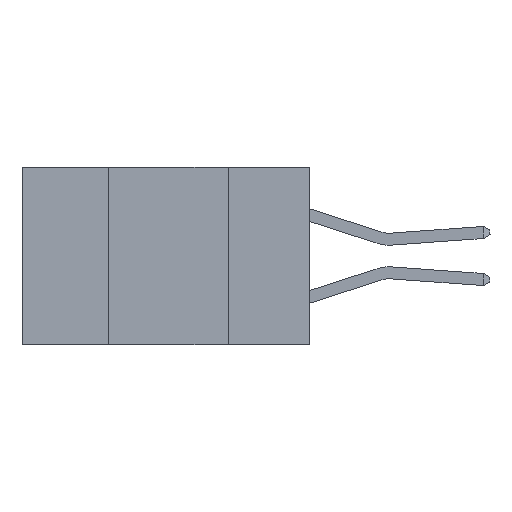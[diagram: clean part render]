
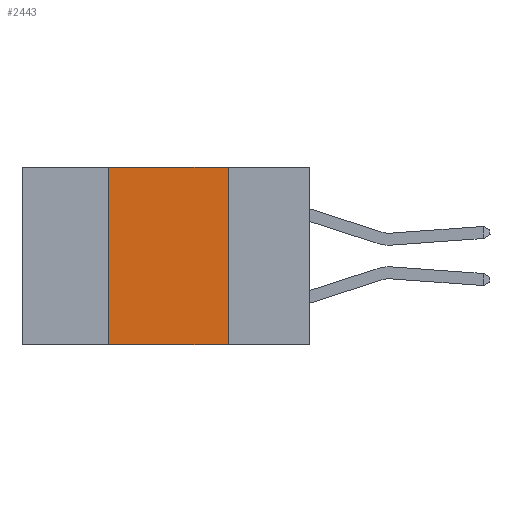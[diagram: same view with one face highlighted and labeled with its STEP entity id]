
A CAD part, left-side view. The second image highlights one B-rep face of the part: STEP entity #2443.
In plain terms, the highlighted planar face has unit normal (-1, 0, 0).
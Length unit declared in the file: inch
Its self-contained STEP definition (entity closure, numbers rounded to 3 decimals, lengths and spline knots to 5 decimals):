
#773 = AXIS2_PLACEMENT_3D ( 'NONE', #8402, #9280, #1180 ) ;
#1180 = DIRECTION ( 'NONE',  ( 0., 0., -1. ) ) ;
#1448 = EDGE_CURVE ( 'NONE', #11548, #8302, #9011, .T. ) ;
#2247 = ORIENTED_EDGE ( 'NONE', *, *, #9435, .F. ) ;
#2373 = ORIENTED_EDGE ( 'NONE', *, *, #10368, .F. ) ;
#2443 = ADVANCED_FACE ( 'NONE', ( #3120 ), #7247, .F. ) ;
#2521 = DIRECTION ( 'NONE',  ( 0., 0., 1. ) ) ;
#3120 = FACE_OUTER_BOUND ( 'NONE', #11360, .T. ) ;
#3586 = VECTOR ( 'NONE', #12138, 39.37008 ) ;
#4204 = LINE ( 'NONE', #10278, #9896 ) ;
#4643 = VERTEX_POINT ( 'NONE', #4987 ) ;
#4974 = EDGE_CURVE ( 'NONE', #11548, #6162, #6574, .T. ) ;
#4987 = CARTESIAN_POINT ( 'NONE',  ( 0., 0.17, 0. ) ) ;
#5178 = CARTESIAN_POINT ( 'NONE',  ( 0., 0.42, -0.37 ) ) ;
#5301 = LINE ( 'NONE', #7387, #7743 ) ;
#5367 = DIRECTION ( 'NONE',  ( 0., -1., 0. ) ) ;
#6162 = VERTEX_POINT ( 'NONE', #11554 ) ;
#6225 = DIRECTION ( 'NONE',  ( 0., 0., -1. ) ) ;
#6574 = LINE ( 'NONE', #8883, #11811 ) ;
#6811 = ORIENTED_EDGE ( 'NONE', *, *, #1448, .T. ) ;
#7247 = PLANE ( 'NONE',  #773 ) ;
#7387 = CARTESIAN_POINT ( 'NONE',  ( 0., 0.6, 0. ) ) ;
#7743 = VECTOR ( 'NONE', #5367, 39.37008 ) ;
#8302 = VERTEX_POINT ( 'NONE', #10230 ) ;
#8402 = CARTESIAN_POINT ( 'NONE',  ( 0., 0.6, 0. ) ) ;
#8740 = ORIENTED_EDGE ( 'NONE', *, *, #4974, .F. ) ;
#8883 = CARTESIAN_POINT ( 'NONE',  ( 0., 0.42, -0.37 ) ) ;
#9011 = LINE ( 'NONE', #13300, #3586 ) ;
#9280 = DIRECTION ( 'NONE',  ( 1., 0., 0. ) ) ;
#9435 = EDGE_CURVE ( 'NONE', #4643, #8302, #4204, .T. ) ;
#9896 = VECTOR ( 'NONE', #6225, 39.37008 ) ;
#10230 = CARTESIAN_POINT ( 'NONE',  ( 0., 0.17, -0.37 ) ) ;
#10278 = CARTESIAN_POINT ( 'NONE',  ( 0., 0.17, -0.37 ) ) ;
#10368 = EDGE_CURVE ( 'NONE', #6162, #4643, #5301, .T. ) ;
#11360 = EDGE_LOOP ( 'NONE', ( #2247, #2373, #8740, #6811 ) ) ;
#11548 = VERTEX_POINT ( 'NONE', #5178 ) ;
#11554 = CARTESIAN_POINT ( 'NONE',  ( 0., 0.42, 0. ) ) ;
#11811 = VECTOR ( 'NONE', #2521, 39.37008 ) ;
#12138 = DIRECTION ( 'NONE',  ( 0., -1., 0. ) ) ;
#13300 = CARTESIAN_POINT ( 'NONE',  ( 0., 0.6, -0.37 ) ) ;
